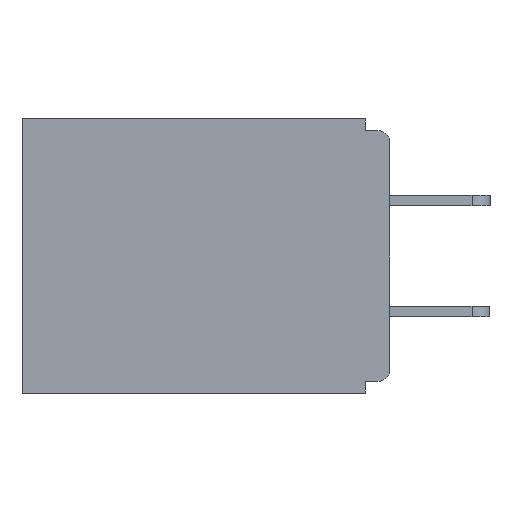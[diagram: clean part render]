
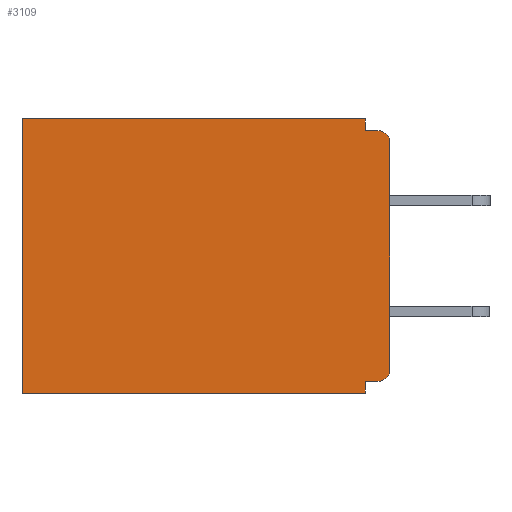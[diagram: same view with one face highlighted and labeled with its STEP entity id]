
A CAD part, left-side view. The second image highlights one B-rep face of the part: STEP entity #3109.
In plain terms, the highlighted planar face has unit normal (-1, 0, 0).
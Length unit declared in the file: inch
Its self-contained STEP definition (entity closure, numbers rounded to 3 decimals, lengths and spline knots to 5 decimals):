
#639 = DIRECTION ( 'NONE',  ( -1., 0., 0. ) ) ;
#793 = ORIENTED_EDGE ( 'NONE', *, *, #3528, .T. ) ;
#818 = EDGE_CURVE ( 'NONE', #13238, #12671, #4267, .T. ) ;
#1202 = CARTESIAN_POINT ( 'NONE',  ( 0.298, 0.46, 0. ) ) ;
#1374 = EDGE_CURVE ( 'NONE', #2959, #6380, #17103, .T. ) ;
#1502 = CARTESIAN_POINT ( 'NONE',  ( 0.298, 0.031, -0.015 ) ) ;
#1692 = ORIENTED_EDGE ( 'NONE', *, *, #1374, .F. ) ;
#1760 = CARTESIAN_POINT ( 'NONE',  ( 0.298, 0., -0.015 ) ) ;
#1843 = ORIENTED_EDGE ( 'NONE', *, *, #6423, .T. ) ;
#1936 = DIRECTION ( 'NONE',  ( 0., 1., 0. ) ) ;
#2359 = CARTESIAN_POINT ( 'NONE',  ( 0.298, 0., -0.343 ) ) ;
#2364 = AXIS2_PLACEMENT_3D ( 'NONE', #10896, #3055, #12363 ) ;
#2736 = DIRECTION ( 'NONE',  ( 0., 0., -1. ) ) ;
#2959 = VERTEX_POINT ( 'NONE', #6770 ) ;
#3048 = DIRECTION ( 'NONE',  ( 0., 0., -1. ) ) ;
#3055 = DIRECTION ( 'NONE',  ( -1., 0., 0. ) ) ;
#3109 = ADVANCED_FACE ( 'NONE', ( #4836 ), #7750, .F. ) ;
#3298 = VERTEX_POINT ( 'NONE', #10749 ) ;
#3528 = EDGE_CURVE ( 'NONE', #15570, #3298, #11687, .T. ) ;
#3557 = VERTEX_POINT ( 'NONE', #6762 ) ;
#3796 = ORIENTED_EDGE ( 'NONE', *, *, #11985, .F. ) ;
#3804 = DIRECTION ( 'NONE',  ( 1., 0., 0. ) ) ;
#3878 = DIRECTION ( 'NONE',  ( 0., 0., -1. ) ) ;
#4252 = VECTOR ( 'NONE', #3878, 39.37008 ) ;
#4267 = LINE ( 'NONE', #10676, #14051 ) ;
#4836 = FACE_OUTER_BOUND ( 'NONE', #6125, .T. ) ;
#5048 = CARTESIAN_POINT ( 'NONE',  ( 0.298, 0.031, 0. ) ) ;
#5056 = EDGE_CURVE ( 'NONE', #5480, #15570, #6035, .T. ) ;
#5480 = VERTEX_POINT ( 'NONE', #5048 ) ;
#5581 = LINE ( 'NONE', #2359, #11008 ) ;
#5763 = ORIENTED_EDGE ( 'NONE', *, *, #16905, .F. ) ;
#5805 = ORIENTED_EDGE ( 'NONE', *, *, #818, .F. ) ;
#6027 = ORIENTED_EDGE ( 'NONE', *, *, #12721, .F. ) ;
#6035 = LINE ( 'NONE', #10421, #16466 ) ;
#6125 = EDGE_LOOP ( 'NONE', ( #13781, #5763, #3796, #14635, #793, #7144, #1692, #6027, #1843, #5805 ) ) ;
#6380 = VERTEX_POINT ( 'NONE', #7217 ) ;
#6423 = EDGE_CURVE ( 'NONE', #15363, #12671, #12928, .T. ) ;
#6762 = CARTESIAN_POINT ( 'NONE',  ( 0.298, 0.015, -0.015 ) ) ;
#6770 = CARTESIAN_POINT ( 'NONE',  ( 0.298, 0.031, -0.328 ) ) ;
#7012 = VECTOR ( 'NONE', #15156, 39.37008 ) ;
#7017 = CARTESIAN_POINT ( 'NONE',  ( 0.298, 0.031, -0.343 ) ) ;
#7144 = ORIENTED_EDGE ( 'NONE', *, *, #16064, .F. ) ;
#7217 = CARTESIAN_POINT ( 'NONE',  ( 0.298, 0.031, -0.343 ) ) ;
#7750 = PLANE ( 'NONE',  #10339 ) ;
#7766 = CARTESIAN_POINT ( 'NONE',  ( 0.298, 0.015, -0.328 ) ) ;
#9742 = EDGE_CURVE ( 'NONE', #13238, #3557, #14090, .T. ) ;
#10339 = AXIS2_PLACEMENT_3D ( 'NONE', #11869, #3804, #17117 ) ;
#10421 = CARTESIAN_POINT ( 'NONE',  ( 0.298, 0., 0. ) ) ;
#10521 = LINE ( 'NONE', #7017, #11352 ) ;
#10633 = DIRECTION ( 'NONE',  ( 0., 1., 0. ) ) ;
#10676 = CARTESIAN_POINT ( 'NONE',  ( 0.298, 0., 0. ) ) ;
#10749 = CARTESIAN_POINT ( 'NONE',  ( 0.298, 0.46, -0.343 ) ) ;
#10896 = CARTESIAN_POINT ( 'NONE',  ( 0.298, 0.015, -0.03 ) ) ;
#11008 = VECTOR ( 'NONE', #16993, 39.37008 ) ;
#11352 = VECTOR ( 'NONE', #3048, 39.37008 ) ;
#11687 = LINE ( 'NONE', #1202, #16205 ) ;
#11824 = CARTESIAN_POINT ( 'NONE',  ( 0.298, 0.031, -0.343 ) ) ;
#11869 = CARTESIAN_POINT ( 'NONE',  ( 0.298, 0., 0. ) ) ;
#11985 = EDGE_CURVE ( 'NONE', #5480, #13763, #10521, .T. ) ;
#12099 = DIRECTION ( 'NONE',  ( 0., 0., -1. ) ) ;
#12363 = DIRECTION ( 'NONE',  ( 0., 0., -1. ) ) ;
#12671 = VERTEX_POINT ( 'NONE', #13282 ) ;
#12678 = DIRECTION ( 'NONE',  ( 0., 0., -1. ) ) ;
#12721 = EDGE_CURVE ( 'NONE', #15363, #2959, #16319, .T. ) ;
#12829 = VECTOR ( 'NONE', #10633, 39.37008 ) ;
#12928 = CIRCLE ( 'NONE', #14377, 0.015 ) ;
#13238 = VERTEX_POINT ( 'NONE', #16666 ) ;
#13282 = CARTESIAN_POINT ( 'NONE',  ( 0.298, 0., -0.313 ) ) ;
#13329 = CARTESIAN_POINT ( 'NONE',  ( 0.298, 0., -0.328 ) ) ;
#13763 = VERTEX_POINT ( 'NONE', #1502 ) ;
#13770 = CARTESIAN_POINT ( 'NONE',  ( 0.298, 0.015, -0.313 ) ) ;
#13781 = ORIENTED_EDGE ( 'NONE', *, *, #9742, .T. ) ;
#13789 = CARTESIAN_POINT ( 'NONE',  ( 0.298, 0.46, 0. ) ) ;
#14051 = VECTOR ( 'NONE', #12099, 39.37008 ) ;
#14090 = CIRCLE ( 'NONE', #2364, 0.015 ) ;
#14316 = LINE ( 'NONE', #1760, #7012 ) ;
#14377 = AXIS2_PLACEMENT_3D ( 'NONE', #13770, #639, #12678 ) ;
#14635 = ORIENTED_EDGE ( 'NONE', *, *, #5056, .T. ) ;
#15156 = DIRECTION ( 'NONE',  ( 0., -1., 0. ) ) ;
#15363 = VERTEX_POINT ( 'NONE', #7766 ) ;
#15570 = VERTEX_POINT ( 'NONE', #13789 ) ;
#16064 = EDGE_CURVE ( 'NONE', #6380, #3298, #5581, .T. ) ;
#16205 = VECTOR ( 'NONE', #2736, 39.37008 ) ;
#16319 = LINE ( 'NONE', #13329, #12829 ) ;
#16466 = VECTOR ( 'NONE', #1936, 39.37008 ) ;
#16666 = CARTESIAN_POINT ( 'NONE',  ( 0.298, 0., -0.03 ) ) ;
#16905 = EDGE_CURVE ( 'NONE', #13763, #3557, #14316, .T. ) ;
#16993 = DIRECTION ( 'NONE',  ( 0., 1., 0. ) ) ;
#17103 = LINE ( 'NONE', #11824, #4252 ) ;
#17117 = DIRECTION ( 'NONE',  ( 0., 0., -1. ) ) ;
